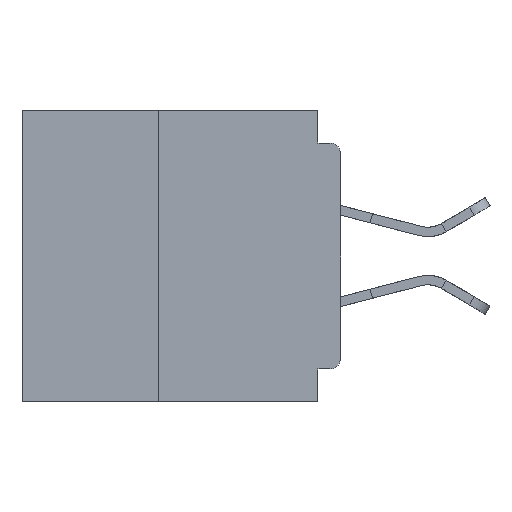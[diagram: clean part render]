
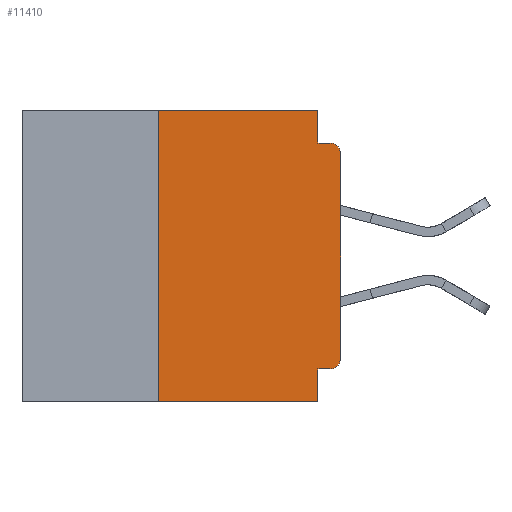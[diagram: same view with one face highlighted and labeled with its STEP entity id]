
A CAD part, left-side view. The second image highlights one B-rep face of the part: STEP entity #11410.
In plain terms, the highlighted planar face has unit normal (-1, 0, 0).
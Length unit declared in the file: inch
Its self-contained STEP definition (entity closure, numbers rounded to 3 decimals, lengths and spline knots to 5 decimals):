
#1186 = CARTESIAN_POINT ( 'NONE',  ( 0., 0.031, -0.355 ) ) ;
#1516 = VERTEX_POINT ( 'NONE', #20299 ) ;
#2403 = ORIENTED_EDGE ( 'NONE', *, *, #26520, .F. ) ;
#2610 = LINE ( 'NONE', #49148, #20467 ) ;
#3258 = CARTESIAN_POINT ( 'NONE',  ( 0., 0.015, -0.06 ) ) ;
#3443 = EDGE_CURVE ( 'NONE', #35187, #17144, #48614, .T. ) ;
#3571 = DIRECTION ( 'NONE',  ( 0., 0., 1. ) ) ;
#4821 = CARTESIAN_POINT ( 'NONE',  ( 0., 0.031, 0. ) ) ;
#6942 = ORIENTED_EDGE ( 'NONE', *, *, #44641, .F. ) ;
#6985 = CARTESIAN_POINT ( 'NONE',  ( 0., 0.031, -0.4 ) ) ;
#7098 = CARTESIAN_POINT ( 'NONE',  ( 0., 0.031, 0. ) ) ;
#7112 = DIRECTION ( 'NONE',  ( 0., 0., -1. ) ) ;
#7281 = VECTOR ( 'NONE', #18224, 39.37008 ) ;
#7360 = CARTESIAN_POINT ( 'NONE',  ( 0., 0., -0.355 ) ) ;
#7830 = VECTOR ( 'NONE', #33723, 39.37008 ) ;
#8019 = FACE_OUTER_BOUND ( 'NONE', #19115, .T. ) ;
#8456 = VECTOR ( 'NONE', #25925, 39.37008 ) ;
#9014 = CARTESIAN_POINT ( 'NONE',  ( 0., 0.437, -0.4 ) ) ;
#9194 = LINE ( 'NONE', #7360, #48366 ) ;
#9653 = LINE ( 'NONE', #6985, #8456 ) ;
#9928 = VECTOR ( 'NONE', #12514, 39.37008 ) ;
#10236 = PLANE ( 'NONE',  #17443 ) ;
#10651 = EDGE_CURVE ( 'NONE', #27303, #27781, #31800, .T. ) ;
#11410 = ADVANCED_FACE ( 'NONE', ( #8019 ), #10236, .F. ) ;
#12300 = CARTESIAN_POINT ( 'NONE',  ( 0., 0., -0.34 ) ) ;
#12514 = DIRECTION ( 'NONE',  ( 0., 0., -1. ) ) ;
#14072 = DIRECTION ( 'NONE',  ( 0., 0., -1. ) ) ;
#14596 = EDGE_CURVE ( 'NONE', #42968, #35395, #29143, .T. ) ;
#15860 = CARTESIAN_POINT ( 'NONE',  ( 0., 0., -0.06 ) ) ;
#16757 = VERTEX_POINT ( 'NONE', #23170 ) ;
#17144 = VERTEX_POINT ( 'NONE', #48168 ) ;
#17286 = EDGE_CURVE ( 'NONE', #27303, #35353, #9194, .T. ) ;
#17443 = AXIS2_PLACEMENT_3D ( 'NONE', #21534, #36810, #14072 ) ;
#17457 = VECTOR ( 'NONE', #3571, 39.37008 ) ;
#18007 = ORIENTED_EDGE ( 'NONE', *, *, #10651, .T. ) ;
#18224 = DIRECTION ( 'NONE',  ( 0., -1., 0. ) ) ;
#19115 = EDGE_LOOP ( 'NONE', ( #40591, #38411, #29042, #2403, #49127, #6942, #26555, #40090, #23950, #18007 ) ) ;
#20025 = LINE ( 'NONE', #4821, #9928 ) ;
#20299 = CARTESIAN_POINT ( 'NONE',  ( 0., 0.031, -0.045 ) ) ;
#20467 = VECTOR ( 'NONE', #45343, 39.37008 ) ;
#21094 = DIRECTION ( 'NONE',  ( -1., 0., 0. ) ) ;
#21534 = CARTESIAN_POINT ( 'NONE',  ( 0., 0.437, 0. ) ) ;
#22043 = CARTESIAN_POINT ( 'NONE',  ( 0., 0.437, 0. ) ) ;
#23170 = CARTESIAN_POINT ( 'NONE',  ( 0., 0.25, 0. ) ) ;
#23603 = EDGE_CURVE ( 'NONE', #35353, #17144, #9653, .T. ) ;
#23950 = ORIENTED_EDGE ( 'NONE', *, *, #17286, .F. ) ;
#25925 = DIRECTION ( 'NONE',  ( 0., 0., -1. ) ) ;
#26520 = EDGE_CURVE ( 'NONE', #35036, #1516, #20025, .T. ) ;
#26555 = ORIENTED_EDGE ( 'NONE', *, *, #3443, .T. ) ;
#27303 = VERTEX_POINT ( 'NONE', #35744 ) ;
#27578 = LINE ( 'NONE', #41546, #17457 ) ;
#27781 = VERTEX_POINT ( 'NONE', #12300 ) ;
#28034 = LINE ( 'NONE', #36717, #7830 ) ;
#28271 = EDGE_CURVE ( 'NONE', #27781, #42968, #27578, .T. ) ;
#29042 = ORIENTED_EDGE ( 'NONE', *, *, #29418, .F. ) ;
#29143 = CIRCLE ( 'NONE', #48648, 0.015 ) ;
#29418 = EDGE_CURVE ( 'NONE', #1516, #35395, #28034, .T. ) ;
#29889 = DIRECTION ( 'NONE',  ( -1., 0., 0. ) ) ;
#31800 = CIRCLE ( 'NONE', #48229, 0.015 ) ;
#33723 = DIRECTION ( 'NONE',  ( 0., -1., 0. ) ) ;
#35036 = VERTEX_POINT ( 'NONE', #7098 ) ;
#35187 = VERTEX_POINT ( 'NONE', #42049 ) ;
#35353 = VERTEX_POINT ( 'NONE', #1186 ) ;
#35395 = VERTEX_POINT ( 'NONE', #35634 ) ;
#35592 = DIRECTION ( 'NONE',  ( 0., -1., 0. ) ) ;
#35634 = CARTESIAN_POINT ( 'NONE',  ( 0., 0.015, -0.045 ) ) ;
#35744 = CARTESIAN_POINT ( 'NONE',  ( 0., 0.015, -0.355 ) ) ;
#36717 = CARTESIAN_POINT ( 'NONE',  ( 0., 0., -0.045 ) ) ;
#36810 = DIRECTION ( 'NONE',  ( 1., 0., 0. ) ) ;
#38411 = ORIENTED_EDGE ( 'NONE', *, *, #14596, .T. ) ;
#38542 = VECTOR ( 'NONE', #35592, 39.37008 ) ;
#40090 = ORIENTED_EDGE ( 'NONE', *, *, #23603, .F. ) ;
#40591 = ORIENTED_EDGE ( 'NONE', *, *, #28271, .T. ) ;
#41546 = CARTESIAN_POINT ( 'NONE',  ( 0., 0., 0. ) ) ;
#42049 = CARTESIAN_POINT ( 'NONE',  ( 0., 0.25, -0.4 ) ) ;
#42968 = VERTEX_POINT ( 'NONE', #15860 ) ;
#43778 = CARTESIAN_POINT ( 'NONE',  ( 0., 0.015, -0.34 ) ) ;
#44641 = EDGE_CURVE ( 'NONE', #35187, #16757, #2610, .T. ) ;
#45318 = DIRECTION ( 'NONE',  ( 0., 1., 0. ) ) ;
#45343 = DIRECTION ( 'NONE',  ( 0., 0., 1. ) ) ;
#45815 = EDGE_CURVE ( 'NONE', #16757, #35036, #47629, .T. ) ;
#47600 = DIRECTION ( 'NONE',  ( 0., 0., -1. ) ) ;
#47629 = LINE ( 'NONE', #22043, #7281 ) ;
#48168 = CARTESIAN_POINT ( 'NONE',  ( 0., 0.031, -0.4 ) ) ;
#48229 = AXIS2_PLACEMENT_3D ( 'NONE', #43778, #21094, #47600 ) ;
#48366 = VECTOR ( 'NONE', #45318, 39.37008 ) ;
#48614 = LINE ( 'NONE', #9014, #38542 ) ;
#48648 = AXIS2_PLACEMENT_3D ( 'NONE', #3258, #29889, #7112 ) ;
#49127 = ORIENTED_EDGE ( 'NONE', *, *, #45815, .F. ) ;
#49148 = CARTESIAN_POINT ( 'NONE',  ( 0., 0.25, -0.4 ) ) ;
